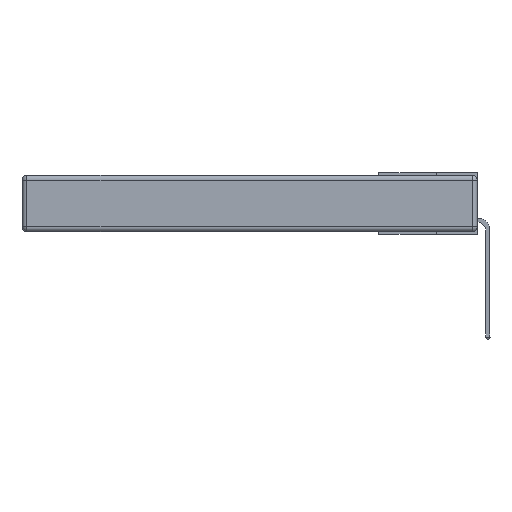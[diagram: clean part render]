
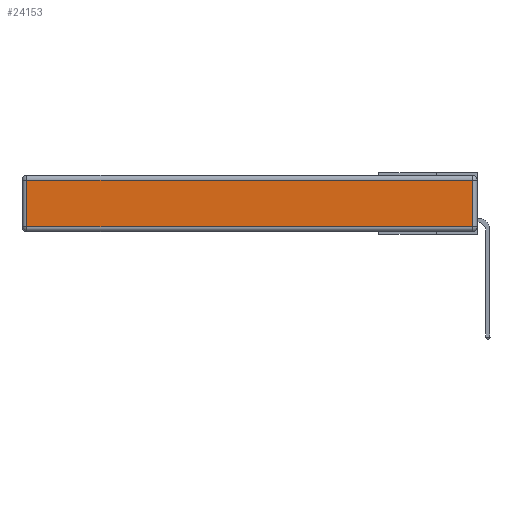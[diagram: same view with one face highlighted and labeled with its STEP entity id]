
A CAD part, left-side view. The second image highlights one B-rep face of the part: STEP entity #24153.
In plain terms, the highlighted planar face has unit normal (-1, 0, 0).
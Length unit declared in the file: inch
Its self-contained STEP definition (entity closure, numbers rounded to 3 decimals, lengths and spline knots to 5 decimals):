
#365 = CARTESIAN_POINT ( 'NONE',  ( 0., 0., -0.343 ) ) ;
#532 = VERTEX_POINT ( 'NONE', #16478 ) ;
#730 = EDGE_CURVE ( 'NONE', #25342, #3246, #26818, .T. ) ;
#1403 = LINE ( 'NONE', #25904, #26692 ) ;
#2230 = DIRECTION ( 'NONE',  ( 0., 0., 1. ) ) ;
#3246 = VERTEX_POINT ( 'NONE', #27115 ) ;
#3741 = FACE_OUTER_BOUND ( 'NONE', #25190, .T. ) ;
#4201 = CARTESIAN_POINT ( 'NONE',  ( 0., 0.03, -0.03 ) ) ;
#4241 = ORIENTED_EDGE ( 'NONE', *, *, #15389, .T. ) ;
#5159 = VECTOR ( 'NONE', #11960, 39.37008 ) ;
#6642 = DIRECTION ( 'NONE',  ( 0., 1., 0. ) ) ;
#8412 = LINE ( 'NONE', #25909, #11137 ) ;
#8800 = DIRECTION ( 'NONE',  ( -1., 0., 0. ) ) ;
#9452 = CARTESIAN_POINT ( 'NONE',  ( 0., 2.72, -0.343 ) ) ;
#11137 = VECTOR ( 'NONE', #6642, 39.37008 ) ;
#11960 = DIRECTION ( 'NONE',  ( 0., -1., 0. ) ) ;
#13189 = CARTESIAN_POINT ( 'NONE',  ( 0., 2.72, -0.313 ) ) ;
#13220 = EDGE_CURVE ( 'NONE', #532, #25342, #21565, .T. ) ;
#13816 = DIRECTION ( 'NONE',  ( 0., 0., -1. ) ) ;
#14689 = AXIS2_PLACEMENT_3D ( 'NONE', #365, #8800, #19736 ) ;
#14830 = EDGE_CURVE ( 'NONE', #3246, #17252, #1403, .T. ) ;
#15389 = EDGE_CURVE ( 'NONE', #17252, #532, #8412, .T. ) ;
#16478 = CARTESIAN_POINT ( 'NONE',  ( 0., 2.72, -0.03 ) ) ;
#17252 = VERTEX_POINT ( 'NONE', #4201 ) ;
#17672 = PLANE ( 'NONE',  #14689 ) ;
#19536 = VECTOR ( 'NONE', #13816, 39.37008 ) ;
#19736 = DIRECTION ( 'NONE',  ( 0., 0., 1. ) ) ;
#20764 = ORIENTED_EDGE ( 'NONE', *, *, #13220, .T. ) ;
#20952 = ORIENTED_EDGE ( 'NONE', *, *, #730, .T. ) ;
#21565 = LINE ( 'NONE', #9452, #19536 ) ;
#24153 = ADVANCED_FACE ( 'NONE', ( #3741 ), #17672, .T. ) ;
#25190 = EDGE_LOOP ( 'NONE', ( #20952, #27072, #4241, #20764 ) ) ;
#25342 = VERTEX_POINT ( 'NONE', #13189 ) ;
#25904 = CARTESIAN_POINT ( 'NONE',  ( 0., 0.03, -0.343 ) ) ;
#25909 = CARTESIAN_POINT ( 'NONE',  ( 0., 2.75, -0.03 ) ) ;
#26692 = VECTOR ( 'NONE', #2230, 39.37008 ) ;
#26818 = LINE ( 'NONE', #27036, #5159 ) ;
#27036 = CARTESIAN_POINT ( 'NONE',  ( 0., 0., -0.313 ) ) ;
#27072 = ORIENTED_EDGE ( 'NONE', *, *, #14830, .T. ) ;
#27115 = CARTESIAN_POINT ( 'NONE',  ( 0., 0.03, -0.313 ) ) ;
